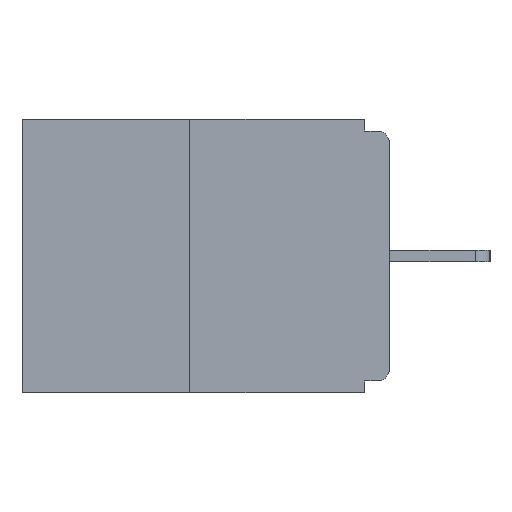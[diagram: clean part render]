
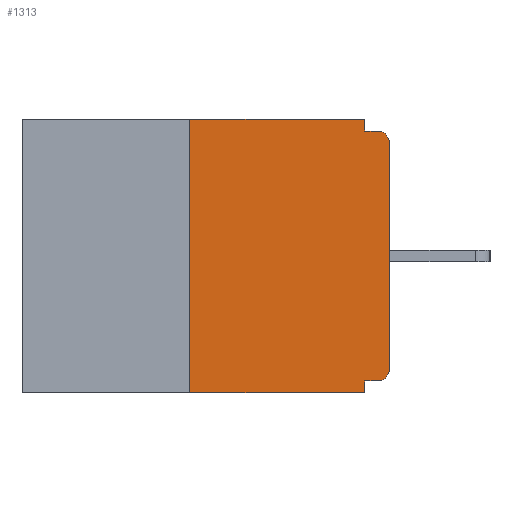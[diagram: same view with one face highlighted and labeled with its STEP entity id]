
A CAD part, left-side view. The second image highlights one B-rep face of the part: STEP entity #1313.
In plain terms, the highlighted planar face has unit normal (-1, 0, 0).
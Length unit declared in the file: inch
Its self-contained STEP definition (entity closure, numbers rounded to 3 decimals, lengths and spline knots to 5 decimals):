
#16 = CARTESIAN_POINT ( 'NONE',  ( 0., 0.031, -0.015 ) ) ;
#112 = EDGE_CURVE ( 'NONE', #4052, #12798, #13584, .T. ) ;
#356 = FACE_OUTER_BOUND ( 'NONE', #8556, .T. ) ;
#373 = VECTOR ( 'NONE', #4162, 39.37008 ) ;
#411 = CARTESIAN_POINT ( 'NONE',  ( 0., 0., -0.328 ) ) ;
#429 = CARTESIAN_POINT ( 'NONE',  ( 0., 0., -0.015 ) ) ;
#579 = ORIENTED_EDGE ( 'NONE', *, *, #4409, .F. ) ;
#698 = DIRECTION ( 'NONE',  ( 0., 0., 1. ) ) ;
#1110 = DIRECTION ( 'NONE',  ( 0., 0., 1. ) ) ;
#1127 = ORIENTED_EDGE ( 'NONE', *, *, #10921, .F. ) ;
#1313 = ADVANCED_FACE ( 'NONE', ( #356 ), #12123, .F. ) ;
#1347 = VERTEX_POINT ( 'NONE', #6228 ) ;
#1376 = EDGE_CURVE ( 'NONE', #13197, #10872, #9867, .T. ) ;
#1539 = VECTOR ( 'NONE', #11020, 39.37008 ) ;
#1677 = LINE ( 'NONE', #3014, #1539 ) ;
#1793 = LINE ( 'NONE', #4125, #8371 ) ;
#1809 = CARTESIAN_POINT ( 'NONE',  ( 0., 0.25, 0. ) ) ;
#1832 = CARTESIAN_POINT ( 'NONE',  ( 0., 0.031, -0.343 ) ) ;
#1923 = EDGE_CURVE ( 'NONE', #13011, #10872, #6488, .T. ) ;
#2056 = CARTESIAN_POINT ( 'NONE',  ( 0., 0.015, -0.03 ) ) ;
#2795 = CARTESIAN_POINT ( 'NONE',  ( 0., 0.46, 0. ) ) ;
#3014 = CARTESIAN_POINT ( 'NONE',  ( 0., 0.46, 0. ) ) ;
#3580 = EDGE_CURVE ( 'NONE', #1347, #14342, #1677, .T. ) ;
#3684 = VECTOR ( 'NONE', #5257, 39.37008 ) ;
#3884 = DIRECTION ( 'NONE',  ( 0., 0., -1. ) ) ;
#3920 = DIRECTION ( 'NONE',  ( -1., 0., 0. ) ) ;
#4052 = VERTEX_POINT ( 'NONE', #15124 ) ;
#4088 = LINE ( 'NONE', #6505, #373 ) ;
#4125 = CARTESIAN_POINT ( 'NONE',  ( 0., 0.031, 0. ) ) ;
#4162 = DIRECTION ( 'NONE',  ( 0., -1., 0. ) ) ;
#4294 = DIRECTION ( 'NONE',  ( 0., 0., -1. ) ) ;
#4317 = VERTEX_POINT ( 'NONE', #13617 ) ;
#4409 = EDGE_CURVE ( 'NONE', #14342, #13197, #1793, .T. ) ;
#4759 = ORIENTED_EDGE ( 'NONE', *, *, #9937, .T. ) ;
#4864 = VERTEX_POINT ( 'NONE', #6599 ) ;
#5183 = VECTOR ( 'NONE', #5196, 39.37008 ) ;
#5196 = DIRECTION ( 'NONE',  ( 0., -1., 0. ) ) ;
#5257 = DIRECTION ( 'NONE',  ( 0., 1., 0. ) ) ;
#5689 = DIRECTION ( 'NONE',  ( 0., 0., -1. ) ) ;
#5884 = ORIENTED_EDGE ( 'NONE', *, *, #112, .F. ) ;
#5940 = LINE ( 'NONE', #10694, #8377 ) ;
#6228 = CARTESIAN_POINT ( 'NONE',  ( 0., 0.25, 0. ) ) ;
#6368 = DIRECTION ( 'NONE',  ( 1., 0., 0. ) ) ;
#6488 = CIRCLE ( 'NONE', #12956, 0.015 ) ;
#6505 = CARTESIAN_POINT ( 'NONE',  ( 0., 0.46, -0.343 ) ) ;
#6518 = VERTEX_POINT ( 'NONE', #8678 ) ;
#6587 = LINE ( 'NONE', #411, #3684 ) ;
#6599 = CARTESIAN_POINT ( 'NONE',  ( 0., 0., -0.313 ) ) ;
#7200 = EDGE_CURVE ( 'NONE', #4317, #1347, #12459, .T. ) ;
#8331 = VECTOR ( 'NONE', #9056, 39.37008 ) ;
#8371 = VECTOR ( 'NONE', #4294, 39.37008 ) ;
#8377 = VECTOR ( 'NONE', #1110, 39.37008 ) ;
#8412 = EDGE_CURVE ( 'NONE', #4317, #12798, #4088, .T. ) ;
#8556 = EDGE_LOOP ( 'NONE', ( #11126, #14295, #8646, #5884, #1127, #10267, #4759, #14909, #11351, #579 ) ) ;
#8646 = ORIENTED_EDGE ( 'NONE', *, *, #8412, .T. ) ;
#8654 = CARTESIAN_POINT ( 'NONE',  ( 0., 0.015, -0.313 ) ) ;
#8678 = CARTESIAN_POINT ( 'NONE',  ( 0., 0.015, -0.328 ) ) ;
#9056 = DIRECTION ( 'NONE',  ( 0., 0., -1. ) ) ;
#9162 = VECTOR ( 'NONE', #698, 39.37008 ) ;
#9269 = AXIS2_PLACEMENT_3D ( 'NONE', #2795, #6368, #3884 ) ;
#9867 = LINE ( 'NONE', #429, #5183 ) ;
#9937 = EDGE_CURVE ( 'NONE', #4864, #13011, #5940, .T. ) ;
#10065 = EDGE_CURVE ( 'NONE', #6518, #4864, #13857, .T. ) ;
#10082 = CARTESIAN_POINT ( 'NONE',  ( 0., 0., -0.03 ) ) ;
#10267 = ORIENTED_EDGE ( 'NONE', *, *, #10065, .T. ) ;
#10596 = DIRECTION ( 'NONE',  ( -1., 0., 0. ) ) ;
#10694 = CARTESIAN_POINT ( 'NONE',  ( 0., 0., 0. ) ) ;
#10872 = VERTEX_POINT ( 'NONE', #13750 ) ;
#10921 = EDGE_CURVE ( 'NONE', #6518, #4052, #6587, .T. ) ;
#11020 = DIRECTION ( 'NONE',  ( 0., -1., 0. ) ) ;
#11126 = ORIENTED_EDGE ( 'NONE', *, *, #3580, .F. ) ;
#11137 = DIRECTION ( 'NONE',  ( 0., 0., -1. ) ) ;
#11351 = ORIENTED_EDGE ( 'NONE', *, *, #1376, .F. ) ;
#12123 = PLANE ( 'NONE',  #9269 ) ;
#12344 = AXIS2_PLACEMENT_3D ( 'NONE', #8654, #3920, #11137 ) ;
#12459 = LINE ( 'NONE', #1809, #9162 ) ;
#12798 = VERTEX_POINT ( 'NONE', #13073 ) ;
#12956 = AXIS2_PLACEMENT_3D ( 'NONE', #2056, #10596, #5689 ) ;
#13011 = VERTEX_POINT ( 'NONE', #10082 ) ;
#13073 = CARTESIAN_POINT ( 'NONE',  ( 0., 0.031, -0.343 ) ) ;
#13197 = VERTEX_POINT ( 'NONE', #16 ) ;
#13584 = LINE ( 'NONE', #1832, #8331 ) ;
#13617 = CARTESIAN_POINT ( 'NONE',  ( 0., 0.25, -0.343 ) ) ;
#13750 = CARTESIAN_POINT ( 'NONE',  ( 0., 0.015, -0.015 ) ) ;
#13857 = CIRCLE ( 'NONE', #12344, 0.015 ) ;
#14156 = CARTESIAN_POINT ( 'NONE',  ( 0., 0.031, 0. ) ) ;
#14295 = ORIENTED_EDGE ( 'NONE', *, *, #7200, .F. ) ;
#14342 = VERTEX_POINT ( 'NONE', #14156 ) ;
#14909 = ORIENTED_EDGE ( 'NONE', *, *, #1923, .T. ) ;
#15124 = CARTESIAN_POINT ( 'NONE',  ( 0., 0.031, -0.328 ) ) ;
